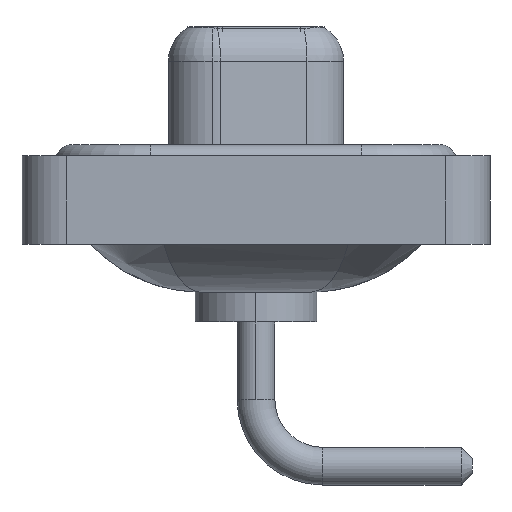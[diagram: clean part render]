
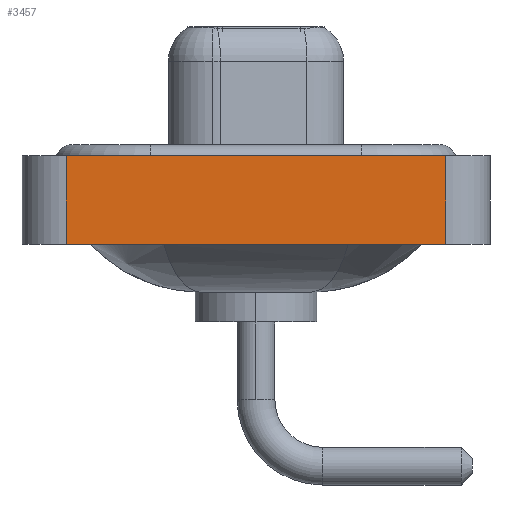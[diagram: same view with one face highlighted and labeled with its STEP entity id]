
A CAD part, left-side view. The second image highlights one B-rep face of the part: STEP entity #3457.
In plain terms, the highlighted planar face has unit normal (-1, 0, 0).
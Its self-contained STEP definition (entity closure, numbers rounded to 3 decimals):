
#338 = CARTESIAN_POINT ( 'NONE',  ( -7.3, -8.55, -3.6 ) ) ;
#607 = VERTEX_POINT ( 'NONE', #338 ) ;
#610 = AXIS2_PLACEMENT_3D ( 'NONE', #6281, #13811, #12613 ) ;
#718 = CARTESIAN_POINT ( 'NONE',  ( -7.3, 8.55, -3.6 ) ) ;
#2248 = VECTOR ( 'NONE', #7129, 1000. ) ;
#2498 = FACE_OUTER_BOUND ( 'NONE', #7790, .T. ) ;
#2517 = VECTOR ( 'NONE', #2518, 1000. ) ;
#2518 = DIRECTION ( 'NONE',  ( 0., 0., 1. ) ) ;
#2814 = VERTEX_POINT ( 'NONE', #11682 ) ;
#2834 = ORIENTED_EDGE ( 'NONE', *, *, #14135, .T. ) ;
#2902 = LINE ( 'NONE', #6463, #11237 ) ;
#2981 = EDGE_CURVE ( 'NONE', #10883, #4945, #9821, .T. ) ;
#3101 = EDGE_CURVE ( 'NONE', #607, #2814, #14812, .T. ) ;
#3457 = ADVANCED_FACE ( 'NONE', ( #2498 ), #12536, .T. ) ;
#3962 = DIRECTION ( 'NONE',  ( 0., -1., 0. ) ) ;
#4848 = CARTESIAN_POINT ( 'NONE',  ( -7.3, 8.55, -3.6 ) ) ;
#4945 = VERTEX_POINT ( 'NONE', #7594 ) ;
#5792 = LINE ( 'NONE', #12136, #14635 ) ;
#5872 = DIRECTION ( 'NONE',  ( 0., -1., 0. ) ) ;
#6281 = CARTESIAN_POINT ( 'NONE',  ( -7.3, -8.55, -3.6 ) ) ;
#6463 = CARTESIAN_POINT ( 'NONE',  ( -7.3, -8.55, 0.4 ) ) ;
#6767 = EDGE_CURVE ( 'NONE', #4945, #2814, #2902, .T. ) ;
#7129 = DIRECTION ( 'NONE',  ( 0., 0., 1. ) ) ;
#7594 = CARTESIAN_POINT ( 'NONE',  ( -7.3, 8.55, 0.4 ) ) ;
#7790 = EDGE_LOOP ( 'NONE', ( #13430, #8109, #11355, #2834 ) ) ;
#8109 = ORIENTED_EDGE ( 'NONE', *, *, #6767, .F. ) ;
#8671 = CARTESIAN_POINT ( 'NONE',  ( -7.3, -8.55, -3.6 ) ) ;
#9821 = LINE ( 'NONE', #4848, #2248 ) ;
#10883 = VERTEX_POINT ( 'NONE', #718 ) ;
#11237 = VECTOR ( 'NONE', #3962, 1000. ) ;
#11355 = ORIENTED_EDGE ( 'NONE', *, *, #2981, .F. ) ;
#11682 = CARTESIAN_POINT ( 'NONE',  ( -7.3, -8.55, 0.4 ) ) ;
#12136 = CARTESIAN_POINT ( 'NONE',  ( -7.3, -8.55, -3.6 ) ) ;
#12536 = PLANE ( 'NONE',  #610 ) ;
#12613 = DIRECTION ( 'NONE',  ( 0., 0., 1. ) ) ;
#13430 = ORIENTED_EDGE ( 'NONE', *, *, #3101, .T. ) ;
#13811 = DIRECTION ( 'NONE',  ( -1., 0., 0. ) ) ;
#14135 = EDGE_CURVE ( 'NONE', #10883, #607, #5792, .T. ) ;
#14635 = VECTOR ( 'NONE', #5872, 1000. ) ;
#14812 = LINE ( 'NONE', #8671, #2517 ) ;
